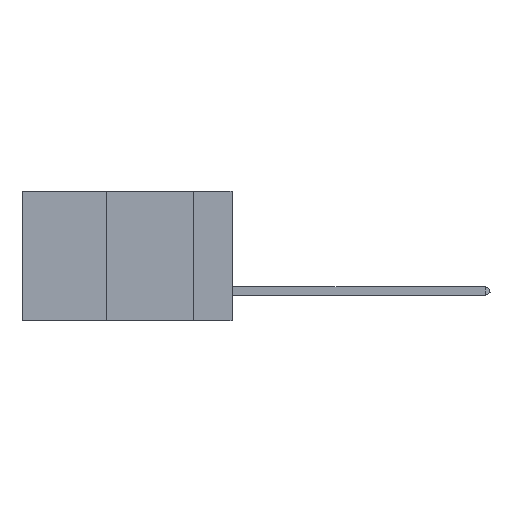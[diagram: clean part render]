
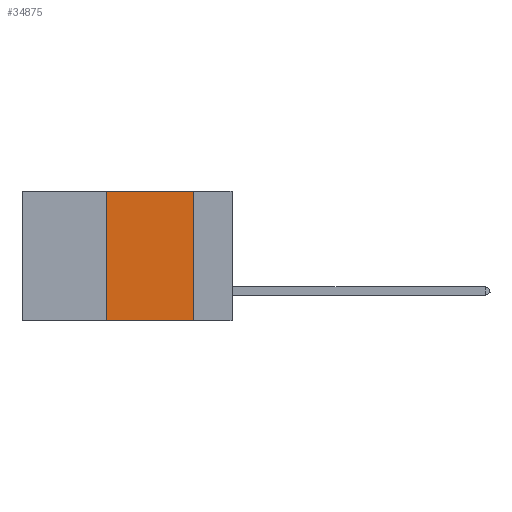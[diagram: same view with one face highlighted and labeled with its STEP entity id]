
A CAD part, left-side view. The second image highlights one B-rep face of the part: STEP entity #34875.
In plain terms, the highlighted planar face has unit normal (-1, 0, 0).
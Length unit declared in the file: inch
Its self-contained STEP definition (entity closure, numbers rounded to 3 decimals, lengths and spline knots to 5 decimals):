
#1542 = VERTEX_POINT ( 'NONE', #26502 ) ;
#1776 = CARTESIAN_POINT ( 'NONE',  ( 0., 0.6, 0. ) ) ;
#4053 = VECTOR ( 'NONE', #43844, 39.37008 ) ;
#4500 = DIRECTION ( 'NONE',  ( 0., -1., 0. ) ) ;
#5946 = ORIENTED_EDGE ( 'NONE', *, *, #14081, .T. ) ;
#8984 = EDGE_CURVE ( 'NONE', #34343, #10215, #38123, .T. ) ;
#9048 = CARTESIAN_POINT ( 'NONE',  ( 0., 0.36, 0. ) ) ;
#10215 = VERTEX_POINT ( 'NONE', #9048 ) ;
#12292 = CARTESIAN_POINT ( 'NONE',  ( 0., 0.6, 0. ) ) ;
#13117 = DIRECTION ( 'NONE',  ( 1., 0., 0. ) ) ;
#13565 = CARTESIAN_POINT ( 'NONE',  ( 0., 0.11, 0. ) ) ;
#14081 = EDGE_CURVE ( 'NONE', #34343, #1542, #41475, .T. ) ;
#14194 = CARTESIAN_POINT ( 'NONE',  ( 0., 0.36, -0.37 ) ) ;
#15225 = EDGE_CURVE ( 'NONE', #10215, #18971, #49883, .T. ) ;
#15423 = VECTOR ( 'NONE', #4500, 39.37008 ) ;
#17191 = PLANE ( 'NONE',  #49972 ) ;
#18971 = VERTEX_POINT ( 'NONE', #13565 ) ;
#19520 = CARTESIAN_POINT ( 'NONE',  ( 0., 0.11, 0. ) ) ;
#20572 = VECTOR ( 'NONE', #35251, 39.37008 ) ;
#23078 = CARTESIAN_POINT ( 'NONE',  ( 0., 0.36, 0. ) ) ;
#26502 = CARTESIAN_POINT ( 'NONE',  ( 0., 0.11, -0.37 ) ) ;
#26943 = VECTOR ( 'NONE', #40000, 39.37008 ) ;
#31912 = CARTESIAN_POINT ( 'NONE',  ( 0., 0.6, -0.37 ) ) ;
#32209 = DIRECTION ( 'NONE',  ( 0., 0., -1. ) ) ;
#34343 = VERTEX_POINT ( 'NONE', #14194 ) ;
#34875 = ADVANCED_FACE ( 'NONE', ( #36361 ), #17191, .F. ) ;
#35251 = DIRECTION ( 'NONE',  ( 0., 0., 1. ) ) ;
#36361 = FACE_OUTER_BOUND ( 'NONE', #47932, .T. ) ;
#36595 = EDGE_CURVE ( 'NONE', #18971, #1542, #44590, .T. ) ;
#38123 = LINE ( 'NONE', #23078, #20572 ) ;
#38746 = ORIENTED_EDGE ( 'NONE', *, *, #8984, .F. ) ;
#39162 = ORIENTED_EDGE ( 'NONE', *, *, #36595, .F. ) ;
#40000 = DIRECTION ( 'NONE',  ( 0., -1., 0. ) ) ;
#40248 = ORIENTED_EDGE ( 'NONE', *, *, #15225, .F. ) ;
#41475 = LINE ( 'NONE', #31912, #26943 ) ;
#43844 = DIRECTION ( 'NONE',  ( 0., 0., -1. ) ) ;
#44590 = LINE ( 'NONE', #19520, #4053 ) ;
#47932 = EDGE_LOOP ( 'NONE', ( #39162, #40248, #38746, #5946 ) ) ;
#49883 = LINE ( 'NONE', #12292, #15423 ) ;
#49972 = AXIS2_PLACEMENT_3D ( 'NONE', #1776, #13117, #32209 ) ;
